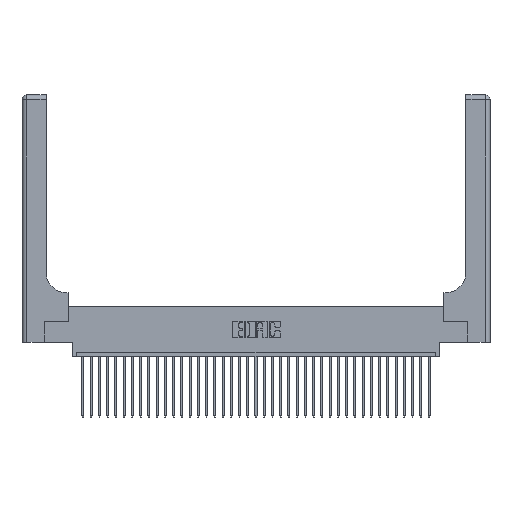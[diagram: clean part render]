
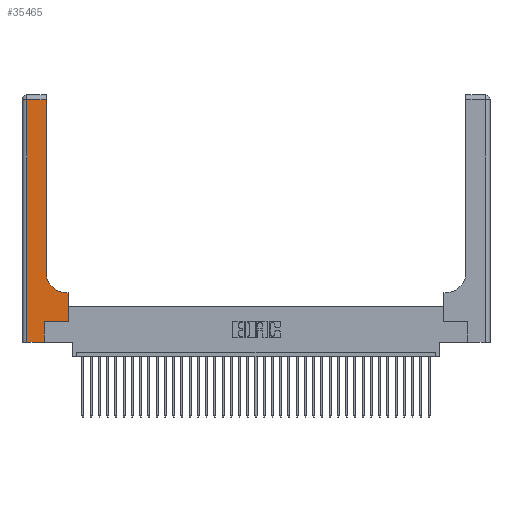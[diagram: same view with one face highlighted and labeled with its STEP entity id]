
A CAD part, top view. The second image highlights one B-rep face of the part: STEP entity #35465.
In plain terms, the highlighted planar face has unit normal (0, 0, 1).
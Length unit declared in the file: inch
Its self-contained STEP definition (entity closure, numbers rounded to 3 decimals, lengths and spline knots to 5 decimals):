
#16 = VERTEX_POINT ( 'NONE', #1651 ) ;
#365 = CARTESIAN_POINT ( 'NONE',  ( 0.269, 0.25, 0.37 ) ) ;
#516 = CARTESIAN_POINT ( 'NONE',  ( 0.2915, 0.6, 0.37 ) ) ;
#555 = CARTESIAN_POINT ( 'NONE',  ( 0., 2.94, 0.37 ) ) ;
#1114 = DIRECTION ( 'NONE',  ( 0., 0., -1. ) ) ;
#1185 = CARTESIAN_POINT ( 'NONE',  ( 0.5585, 0.6, 0.37 ) ) ;
#1651 = CARTESIAN_POINT ( 'NONE',  ( 0.5415, 0.6, 0.37 ) ) ;
#1970 = CARTESIAN_POINT ( 'NONE',  ( 0.269, 0., 0.37 ) ) ;
#2335 = VECTOR ( 'NONE', #15542, 39.37008 ) ;
#2407 = ORIENTED_EDGE ( 'NONE', *, *, #13427, .T. ) ;
#2645 = DIRECTION ( 'NONE',  ( 1., 0., 0. ) ) ;
#2715 = EDGE_CURVE ( 'NONE', #37356, #21386, #36235, .T. ) ;
#3012 = LINE ( 'NONE', #28501, #35170 ) ;
#3037 = VERTEX_POINT ( 'NONE', #22151 ) ;
#4190 = VERTEX_POINT ( 'NONE', #5431 ) ;
#4418 = CARTESIAN_POINT ( 'NONE',  ( 0., 3., 0.37 ) ) ;
#4524 = ORIENTED_EDGE ( 'NONE', *, *, #2715, .T. ) ;
#5431 = CARTESIAN_POINT ( 'NONE',  ( 0.269, 0.25, 0.37 ) ) ;
#6715 = ORIENTED_EDGE ( 'NONE', *, *, #16865, .T. ) ;
#6819 = DIRECTION ( 'NONE',  ( -1., 0., 0. ) ) ;
#7457 = EDGE_CURVE ( 'NONE', #21386, #18768, #23818, .T. ) ;
#8265 = LINE ( 'NONE', #30838, #13710 ) ;
#8452 = CARTESIAN_POINT ( 'NONE',  ( 0.5415, 0.85, 0.37 ) ) ;
#9191 = FACE_OUTER_BOUND ( 'NONE', #16458, .T. ) ;
#9902 = EDGE_CURVE ( 'NONE', #34560, #30625, #37493, .T. ) ;
#9905 = DIRECTION ( 'NONE',  ( 1., 0., 0. ) ) ;
#10003 = LINE ( 'NONE', #27041, #2335 ) ;
#13295 = ORIENTED_EDGE ( 'NONE', *, *, #7457, .T. ) ;
#13427 = EDGE_CURVE ( 'NONE', #18768, #34560, #8265, .T. ) ;
#13487 = DIRECTION ( 'NONE',  ( 0., -1., 0. ) ) ;
#13710 = VECTOR ( 'NONE', #13487, 39.37008 ) ;
#14154 = DIRECTION ( 'NONE',  ( 0., 0., -1. ) ) ;
#14485 = ORIENTED_EDGE ( 'NONE', *, *, #19525, .T. ) ;
#14738 = ORIENTED_EDGE ( 'NONE', *, *, #20756, .T. ) ;
#15542 = DIRECTION ( 'NONE',  ( 0., 1., 0. ) ) ;
#15655 = CARTESIAN_POINT ( 'NONE',  ( 0.2915, 2.94, 0.37 ) ) ;
#16458 = EDGE_LOOP ( 'NONE', ( #4524, #13295, #2407, #23457, #19988, #6715, #14738, #14485, #33664 ) ) ;
#16858 = CARTESIAN_POINT ( 'NONE',  ( 0.06, 0., 0.37 ) ) ;
#16865 = EDGE_CURVE ( 'NONE', #4190, #3037, #17079, .T. ) ;
#17079 = LINE ( 'NONE', #365, #27483 ) ;
#17649 = CIRCLE ( 'NONE', #34051, 0.25 ) ;
#18078 = CARTESIAN_POINT ( 'NONE',  ( 0.2915, 0.85, 0.37 ) ) ;
#18191 = DIRECTION ( 'NONE',  ( 0., 1., 0. ) ) ;
#18768 = VERTEX_POINT ( 'NONE', #34897 ) ;
#19344 = VECTOR ( 'NONE', #33184, 39.37008 ) ;
#19355 = VECTOR ( 'NONE', #6819, 39.37008 ) ;
#19525 = EDGE_CURVE ( 'NONE', #27946, #16, #36392, .T. ) ;
#19613 = VECTOR ( 'NONE', #20925, 39.37008 ) ;
#19694 = DIRECTION ( 'NONE',  ( 0., 1., 0. ) ) ;
#19988 = ORIENTED_EDGE ( 'NONE', *, *, #25779, .T. ) ;
#20756 = EDGE_CURVE ( 'NONE', #3037, #27946, #10003, .T. ) ;
#20925 = DIRECTION ( 'NONE',  ( -1., 0., 0. ) ) ;
#21386 = VERTEX_POINT ( 'NONE', #15655 ) ;
#22151 = CARTESIAN_POINT ( 'NONE',  ( 0.5585, 0.25, 0.37 ) ) ;
#23457 = ORIENTED_EDGE ( 'NONE', *, *, #9902, .T. ) ;
#23818 = LINE ( 'NONE', #555, #19355 ) ;
#24678 = CARTESIAN_POINT ( 'NONE',  ( 0.2915, 3., 0.37 ) ) ;
#25779 = EDGE_CURVE ( 'NONE', #30625, #4190, #3012, .T. ) ;
#27041 = CARTESIAN_POINT ( 'NONE',  ( 0.5585, 0.25, 0.37 ) ) ;
#27271 = PLANE ( 'NONE',  #37040 ) ;
#27483 = VECTOR ( 'NONE', #9905, 39.37008 ) ;
#27946 = VERTEX_POINT ( 'NONE', #1185 ) ;
#28457 = VECTOR ( 'NONE', #18191, 39.37008 ) ;
#28501 = CARTESIAN_POINT ( 'NONE',  ( 0.269, 0., 0.37 ) ) ;
#30625 = VERTEX_POINT ( 'NONE', #1970 ) ;
#30838 = CARTESIAN_POINT ( 'NONE',  ( 0.06, 3., 0.37 ) ) ;
#32868 = DIRECTION ( 'NONE',  ( -1., 0., 0. ) ) ;
#33057 = CARTESIAN_POINT ( 'NONE',  ( 0., 0., 0.37 ) ) ;
#33184 = DIRECTION ( 'NONE',  ( 1., 0., 0. ) ) ;
#33664 = ORIENTED_EDGE ( 'NONE', *, *, #34008, .T. ) ;
#34008 = EDGE_CURVE ( 'NONE', #16, #37356, #17649, .T. ) ;
#34051 = AXIS2_PLACEMENT_3D ( 'NONE', #8452, #14154, #2645 ) ;
#34560 = VERTEX_POINT ( 'NONE', #16858 ) ;
#34897 = CARTESIAN_POINT ( 'NONE',  ( 0.06, 2.94, 0.37 ) ) ;
#35170 = VECTOR ( 'NONE', #19694, 39.37008 ) ;
#35465 = ADVANCED_FACE ( 'NONE', ( #9191 ), #27271, .F. ) ;
#36235 = LINE ( 'NONE', #24678, #28457 ) ;
#36392 = LINE ( 'NONE', #516, #19613 ) ;
#37040 = AXIS2_PLACEMENT_3D ( 'NONE', #4418, #1114, #32868 ) ;
#37356 = VERTEX_POINT ( 'NONE', #18078 ) ;
#37493 = LINE ( 'NONE', #33057, #19344 ) ;
